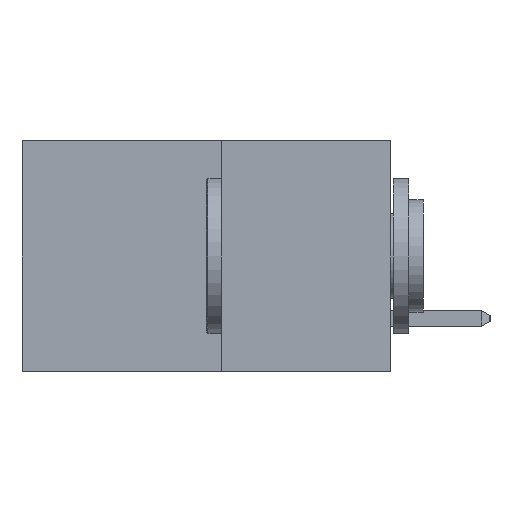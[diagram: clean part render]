
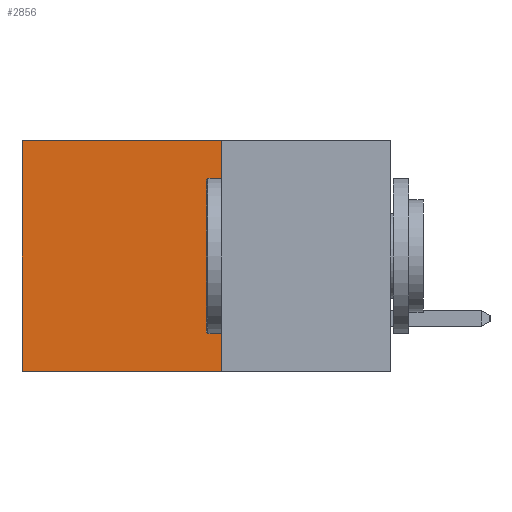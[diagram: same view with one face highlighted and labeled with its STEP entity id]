
A CAD part, left-side view. The second image highlights one B-rep face of the part: STEP entity #2856.
In plain terms, the highlighted planar face has unit normal (-1, 0, 0).
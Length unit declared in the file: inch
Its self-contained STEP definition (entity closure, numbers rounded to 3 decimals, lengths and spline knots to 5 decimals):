
#258 = AXIS2_PLACEMENT_3D ( 'NONE', #3731, #19156, #19098 ) ;
#778 = EDGE_LOOP ( 'NONE', ( #14286, #6672, #12803, #3883 ) ) ;
#2856 = ADVANCED_FACE ( 'NONE', ( #10571 ), #11368, .F. ) ;
#3731 = CARTESIAN_POINT ( 'NONE',  ( 0.277, 0.27, -0.37 ) ) ;
#3883 = ORIENTED_EDGE ( 'NONE', *, *, #18333, .T. ) ;
#4049 = VERTEX_POINT ( 'NONE', #20411 ) ;
#6672 = ORIENTED_EDGE ( 'NONE', *, *, #23378, .F. ) ;
#7051 = CARTESIAN_POINT ( 'NONE',  ( 0.277, 0.59, -0.37 ) ) ;
#7351 = VERTEX_POINT ( 'NONE', #7051 ) ;
#8032 = VECTOR ( 'NONE', #16789, 39.37008 ) ;
#8810 = DIRECTION ( 'NONE',  ( 0., 0., -1. ) ) ;
#8952 = CARTESIAN_POINT ( 'NONE',  ( 0.277, 0.27, 0. ) ) ;
#9595 = CARTESIAN_POINT ( 'NONE',  ( 0.277, 0.27, 0. ) ) ;
#9630 = VECTOR ( 'NONE', #8810, 39.37008 ) ;
#9746 = CARTESIAN_POINT ( 'NONE',  ( 0.277, 0.27, -0.37 ) ) ;
#9754 = VECTOR ( 'NONE', #10962, 39.37008 ) ;
#10114 = EDGE_CURVE ( 'NONE', #4049, #7351, #23530, .T. ) ;
#10246 = LINE ( 'NONE', #14662, #9630 ) ;
#10571 = FACE_OUTER_BOUND ( 'NONE', #778, .T. ) ;
#10962 = DIRECTION ( 'NONE',  ( 0., 1., 0. ) ) ;
#11368 = PLANE ( 'NONE',  #258 ) ;
#12803 = ORIENTED_EDGE ( 'NONE', *, *, #20375, .F. ) ;
#12953 = CARTESIAN_POINT ( 'NONE',  ( 0.277, 0.59, -0.37 ) ) ;
#14286 = ORIENTED_EDGE ( 'NONE', *, *, #10114, .T. ) ;
#14662 = CARTESIAN_POINT ( 'NONE',  ( 0.277, 0.27, -0.37 ) ) ;
#16789 = DIRECTION ( 'NONE',  ( 0., 0., -1. ) ) ;
#17033 = LINE ( 'NONE', #9746, #22115 ) ;
#18153 = VERTEX_POINT ( 'NONE', #23756 ) ;
#18333 = EDGE_CURVE ( 'NONE', #22793, #4049, #20070, .T. ) ;
#19098 = DIRECTION ( 'NONE',  ( 0., 0., -1. ) ) ;
#19156 = DIRECTION ( 'NONE',  ( 1., 0., 0. ) ) ;
#20070 = LINE ( 'NONE', #8952, #9754 ) ;
#20375 = EDGE_CURVE ( 'NONE', #22793, #18153, #10246, .T. ) ;
#20411 = CARTESIAN_POINT ( 'NONE',  ( 0.277, 0.59, 0. ) ) ;
#22115 = VECTOR ( 'NONE', #25192, 39.37008 ) ;
#22793 = VERTEX_POINT ( 'NONE', #9595 ) ;
#23378 = EDGE_CURVE ( 'NONE', #18153, #7351, #17033, .T. ) ;
#23530 = LINE ( 'NONE', #12953, #8032 ) ;
#23756 = CARTESIAN_POINT ( 'NONE',  ( 0.277, 0.27, -0.37 ) ) ;
#25192 = DIRECTION ( 'NONE',  ( 0., 1., 0. ) ) ;
